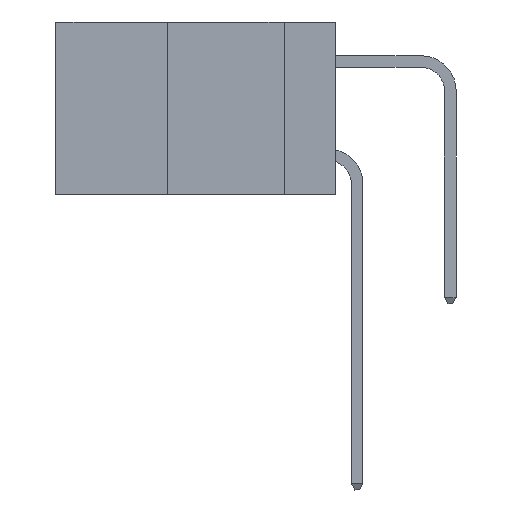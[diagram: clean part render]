
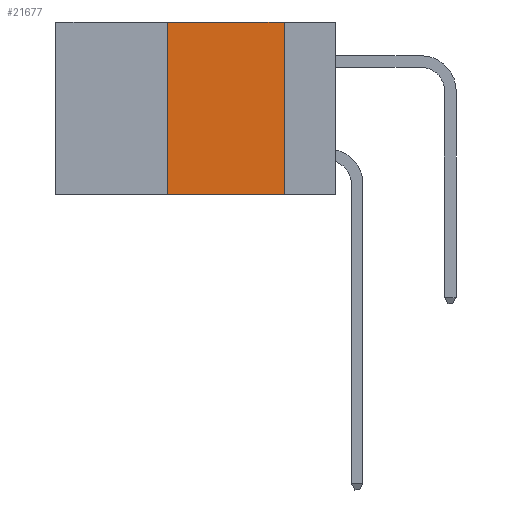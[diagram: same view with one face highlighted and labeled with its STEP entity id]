
A CAD part, left-side view. The second image highlights one B-rep face of the part: STEP entity #21677.
In plain terms, the highlighted planar face has unit normal (-1, 0, 0).
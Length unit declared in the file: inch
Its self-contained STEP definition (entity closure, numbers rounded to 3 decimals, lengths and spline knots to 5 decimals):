
#123 = EDGE_CURVE ( 'NONE', #16504, #45021, #9997, .T. ) ;
#2269 = PLANE ( 'NONE',  #7783 ) ;
#4394 = LINE ( 'NONE', #22605, #29227 ) ;
#5174 = EDGE_CURVE ( 'NONE', #16504, #20242, #38985, .T. ) ;
#7783 = AXIS2_PLACEMENT_3D ( 'NONE', #47935, #29224, #50919 ) ;
#9997 = LINE ( 'NONE', #50935, #38082 ) ;
#12248 = CARTESIAN_POINT ( 'NONE',  ( 0., 0.6, -0.37 ) ) ;
#16504 = VERTEX_POINT ( 'NONE', #28739 ) ;
#17316 = DIRECTION ( 'NONE',  ( 0., 0., 1. ) ) ;
#17318 = ORIENTED_EDGE ( 'NONE', *, *, #30447, .F. ) ;
#18240 = ORIENTED_EDGE ( 'NONE', *, *, #23436, .F. ) ;
#19601 = CARTESIAN_POINT ( 'NONE',  ( 0., 0.36, 0. ) ) ;
#19908 = VERTEX_POINT ( 'NONE', #45441 ) ;
#20242 = VERTEX_POINT ( 'NONE', #27272 ) ;
#21677 = ADVANCED_FACE ( 'NONE', ( #37356 ), #2269, .F. ) ;
#22605 = CARTESIAN_POINT ( 'NONE',  ( 0., 0.11, 0. ) ) ;
#23436 = EDGE_CURVE ( 'NONE', #45021, #19908, #24151, .T. ) ;
#24151 = LINE ( 'NONE', #29442, #38536 ) ;
#25641 = EDGE_LOOP ( 'NONE', ( #17318, #18240, #30420, #51689 ) ) ;
#27272 = CARTESIAN_POINT ( 'NONE',  ( 0., 0.11, -0.37 ) ) ;
#28739 = CARTESIAN_POINT ( 'NONE',  ( 0., 0.36, -0.37 ) ) ;
#29224 = DIRECTION ( 'NONE',  ( 1., 0., 0. ) ) ;
#29227 = VECTOR ( 'NONE', #31177, 39.37008 ) ;
#29442 = CARTESIAN_POINT ( 'NONE',  ( 0., 0.6, 0. ) ) ;
#30154 = DIRECTION ( 'NONE',  ( 0., -1., 0. ) ) ;
#30420 = ORIENTED_EDGE ( 'NONE', *, *, #123, .F. ) ;
#30447 = EDGE_CURVE ( 'NONE', #19908, #20242, #4394, .T. ) ;
#31177 = DIRECTION ( 'NONE',  ( 0., 0., -1. ) ) ;
#37356 = FACE_OUTER_BOUND ( 'NONE', #25641, .T. ) ;
#38082 = VECTOR ( 'NONE', #17316, 39.37008 ) ;
#38536 = VECTOR ( 'NONE', #30154, 39.37008 ) ;
#38985 = LINE ( 'NONE', #12248, #48810 ) ;
#45021 = VERTEX_POINT ( 'NONE', #19601 ) ;
#45441 = CARTESIAN_POINT ( 'NONE',  ( 0., 0.11, 0. ) ) ;
#47935 = CARTESIAN_POINT ( 'NONE',  ( 0., 0.6, 0. ) ) ;
#48810 = VECTOR ( 'NONE', #54133, 39.37008 ) ;
#50919 = DIRECTION ( 'NONE',  ( 0., 0., -1. ) ) ;
#50935 = CARTESIAN_POINT ( 'NONE',  ( 0., 0.36, 0. ) ) ;
#51689 = ORIENTED_EDGE ( 'NONE', *, *, #5174, .T. ) ;
#54133 = DIRECTION ( 'NONE',  ( 0., -1., 0. ) ) ;
